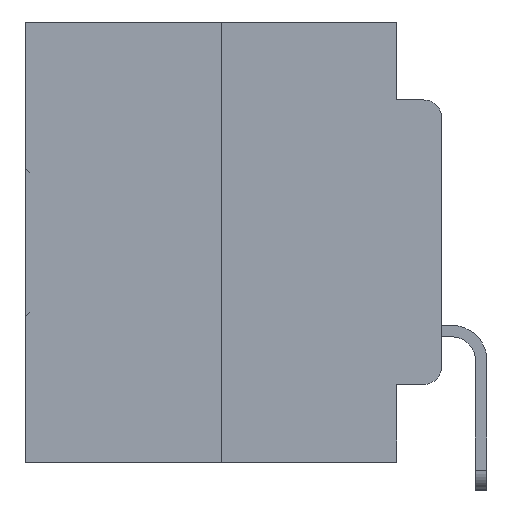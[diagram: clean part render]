
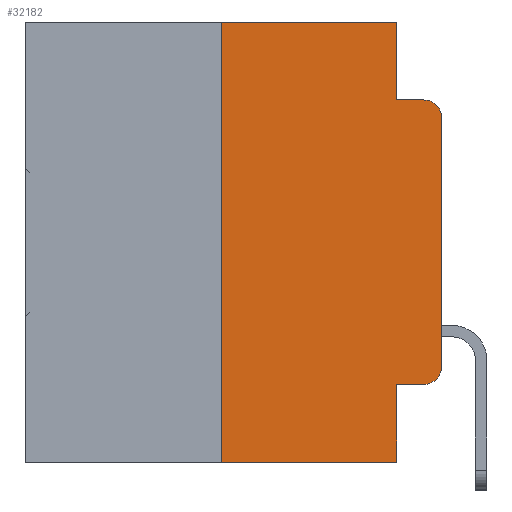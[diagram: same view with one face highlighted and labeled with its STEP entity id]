
A CAD part, left-side view. The second image highlights one B-rep face of the part: STEP entity #32182.
In plain terms, the highlighted planar face has unit normal (-1, 0, 0).
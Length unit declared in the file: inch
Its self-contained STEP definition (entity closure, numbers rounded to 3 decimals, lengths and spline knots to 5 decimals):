
#73 = ORIENTED_EDGE ( 'NONE', *, *, #26438, .T. ) ;
#841 = CARTESIAN_POINT ( 'NONE',  ( 0., 0.02, -0.1085 ) ) ;
#1352 = CARTESIAN_POINT ( 'NONE',  ( 0., 0.051, -0.0885 ) ) ;
#1520 = CARTESIAN_POINT ( 'NONE',  ( 0., 0.25, -0.5 ) ) ;
#2401 = EDGE_LOOP ( 'NONE', ( #29643, #13379, #12935, #29052, #20145, #23115, #20183, #10546, #73, #19676 ) ) ;
#2532 = VECTOR ( 'NONE', #30332, 39.37008 ) ;
#2646 = CARTESIAN_POINT ( 'NONE',  ( 0., 0.051, -0.4115 ) ) ;
#3141 = PLANE ( 'NONE',  #23677 ) ;
#3457 = CARTESIAN_POINT ( 'NONE',  ( 0., 0.02, -0.3915 ) ) ;
#3591 = DIRECTION ( 'NONE',  ( 0., 0., -1. ) ) ;
#4278 = LINE ( 'NONE', #24653, #24590 ) ;
#4590 = VERTEX_POINT ( 'NONE', #2646 ) ;
#4748 = VERTEX_POINT ( 'NONE', #23803 ) ;
#5085 = CARTESIAN_POINT ( 'NONE',  ( 0., 0.02, -0.4115 ) ) ;
#5882 = DIRECTION ( 'NONE',  ( 1., 0., 0. ) ) ;
#6220 = DIRECTION ( 'NONE',  ( 0., 0., -1. ) ) ;
#7066 = DIRECTION ( 'NONE',  ( 0., 0., 1. ) ) ;
#8872 = LINE ( 'NONE', #13274, #2532 ) ;
#9048 = CARTESIAN_POINT ( 'NONE',  ( 0., 0.051, -0.0885 ) ) ;
#10546 = ORIENTED_EDGE ( 'NONE', *, *, #29625, .F. ) ;
#10739 = CARTESIAN_POINT ( 'NONE',  ( 0., 0.473, 0. ) ) ;
#10980 = CARTESIAN_POINT ( 'NONE',  ( 0., 0.473, 0. ) ) ;
#12229 = LINE ( 'NONE', #9048, #30953 ) ;
#12517 = EDGE_CURVE ( 'NONE', #25434, #4748, #8872, .T. ) ;
#12883 = CARTESIAN_POINT ( 'NONE',  ( 0., 0.051, 0. ) ) ;
#12935 = ORIENTED_EDGE ( 'NONE', *, *, #24491, .F. ) ;
#13165 = VECTOR ( 'NONE', #15472, 39.37008 ) ;
#13274 = CARTESIAN_POINT ( 'NONE',  ( 0., 0.473, -0.5 ) ) ;
#13307 = DIRECTION ( 'NONE',  ( 0., -1., 0. ) ) ;
#13321 = VECTOR ( 'NONE', #24607, 39.37008 ) ;
#13379 = ORIENTED_EDGE ( 'NONE', *, *, #27659, .T. ) ;
#15472 = DIRECTION ( 'NONE',  ( 0., 0., -1. ) ) ;
#15848 = LINE ( 'NONE', #21781, #21657 ) ;
#16490 = EDGE_CURVE ( 'NONE', #16714, #26727, #17519, .T. ) ;
#16679 = EDGE_CURVE ( 'NONE', #19935, #27317, #20766, .T. ) ;
#16714 = VERTEX_POINT ( 'NONE', #23911 ) ;
#16745 = VECTOR ( 'NONE', #13307, 39.37008 ) ;
#16906 = DIRECTION ( 'NONE',  ( 0., 0., -1. ) ) ;
#17519 = LINE ( 'NONE', #10739, #16745 ) ;
#17738 = VECTOR ( 'NONE', #21330, 39.37008 ) ;
#17948 = AXIS2_PLACEMENT_3D ( 'NONE', #3457, #21507, #6220 ) ;
#19166 = DIRECTION ( 'NONE',  ( -1., 0., 0. ) ) ;
#19676 = ORIENTED_EDGE ( 'NONE', *, *, #16679, .T. ) ;
#19935 = VERTEX_POINT ( 'NONE', #5085 ) ;
#20101 = FACE_OUTER_BOUND ( 'NONE', #2401, .T. ) ;
#20145 = ORIENTED_EDGE ( 'NONE', *, *, #16490, .F. ) ;
#20183 = ORIENTED_EDGE ( 'NONE', *, *, #12517, .T. ) ;
#20766 = CIRCLE ( 'NONE', #17948, 0.02 ) ;
#20836 = CARTESIAN_POINT ( 'NONE',  ( 0., 0.051, 0. ) ) ;
#21330 = DIRECTION ( 'NONE',  ( 0., 0., 1. ) ) ;
#21467 = VERTEX_POINT ( 'NONE', #25199 ) ;
#21507 = DIRECTION ( 'NONE',  ( -1., 0., 0. ) ) ;
#21657 = VECTOR ( 'NONE', #16906, 39.37008 ) ;
#21781 = CARTESIAN_POINT ( 'NONE',  ( 0., 0.051, 0. ) ) ;
#22216 = CARTESIAN_POINT ( 'NONE',  ( 0., 0.051, -0.4115 ) ) ;
#23115 = ORIENTED_EDGE ( 'NONE', *, *, #32247, .F. ) ;
#23233 = AXIS2_PLACEMENT_3D ( 'NONE', #841, #19166, #3591 ) ;
#23610 = DIRECTION ( 'NONE',  ( 0., 0., -1. ) ) ;
#23677 = AXIS2_PLACEMENT_3D ( 'NONE', #10980, #5882, #23610 ) ;
#23803 = CARTESIAN_POINT ( 'NONE',  ( 0., 0.051, -0.5 ) ) ;
#23911 = CARTESIAN_POINT ( 'NONE',  ( 0., 0.25, 0. ) ) ;
#24491 = EDGE_CURVE ( 'NONE', #29371, #21467, #12229, .T. ) ;
#24590 = VECTOR ( 'NONE', #7066, 39.37008 ) ;
#24607 = DIRECTION ( 'NONE',  ( 0., -1., 0. ) ) ;
#24653 = CARTESIAN_POINT ( 'NONE',  ( 0., 0., 0. ) ) ;
#25199 = CARTESIAN_POINT ( 'NONE',  ( 0., 0.02, -0.0885 ) ) ;
#25434 = VERTEX_POINT ( 'NONE', #1520 ) ;
#26421 = DIRECTION ( 'NONE',  ( 0., -1., 0. ) ) ;
#26438 = EDGE_CURVE ( 'NONE', #4590, #19935, #32742, .T. ) ;
#26727 = VERTEX_POINT ( 'NONE', #20836 ) ;
#27317 = VERTEX_POINT ( 'NONE', #27569 ) ;
#27569 = CARTESIAN_POINT ( 'NONE',  ( 0., 0., -0.3915 ) ) ;
#27659 = EDGE_CURVE ( 'NONE', #31150, #21467, #31533, .T. ) ;
#28582 = CARTESIAN_POINT ( 'NONE',  ( 0., 0.25, 0. ) ) ;
#29052 = ORIENTED_EDGE ( 'NONE', *, *, #31648, .F. ) ;
#29371 = VERTEX_POINT ( 'NONE', #1352 ) ;
#29625 = EDGE_CURVE ( 'NONE', #4590, #4748, #32610, .T. ) ;
#29643 = ORIENTED_EDGE ( 'NONE', *, *, #32491, .T. ) ;
#30332 = DIRECTION ( 'NONE',  ( 0., -1., 0. ) ) ;
#30537 = LINE ( 'NONE', #28582, #17738 ) ;
#30953 = VECTOR ( 'NONE', #26421, 39.37008 ) ;
#31150 = VERTEX_POINT ( 'NONE', #31482 ) ;
#31482 = CARTESIAN_POINT ( 'NONE',  ( 0., 0., -0.1085 ) ) ;
#31533 = CIRCLE ( 'NONE', #23233, 0.02 ) ;
#31648 = EDGE_CURVE ( 'NONE', #26727, #29371, #15848, .T. ) ;
#32182 = ADVANCED_FACE ( 'NONE', ( #20101 ), #3141, .F. ) ;
#32247 = EDGE_CURVE ( 'NONE', #25434, #16714, #30537, .T. ) ;
#32491 = EDGE_CURVE ( 'NONE', #27317, #31150, #4278, .T. ) ;
#32610 = LINE ( 'NONE', #12883, #13165 ) ;
#32742 = LINE ( 'NONE', #22216, #13321 ) ;
